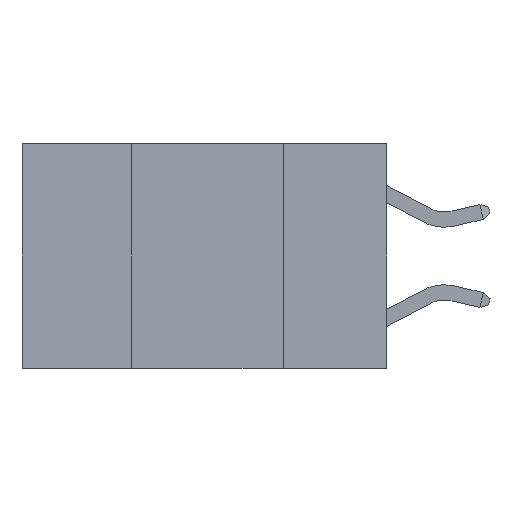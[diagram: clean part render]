
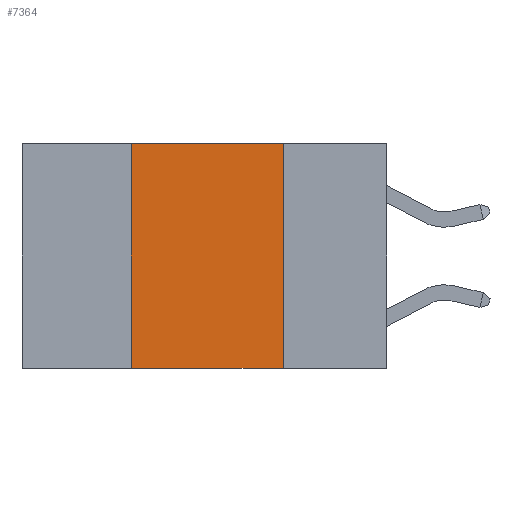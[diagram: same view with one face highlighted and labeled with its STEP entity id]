
A CAD part, left-side view. The second image highlights one B-rep face of the part: STEP entity #7364.
In plain terms, the highlighted planar face has unit normal (-1, 0, 0).
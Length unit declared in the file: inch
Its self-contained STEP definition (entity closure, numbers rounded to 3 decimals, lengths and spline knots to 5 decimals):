
#1609 = VECTOR ( 'NONE', #2965, 39.37008 ) ;
#1902 = CARTESIAN_POINT ( 'NONE',  ( 0., 0.17, 0. ) ) ;
#1964 = PLANE ( 'NONE',  #10545 ) ;
#2076 = LINE ( 'NONE', #8382, #9908 ) ;
#2579 = LINE ( 'NONE', #5825, #6420 ) ;
#2965 = DIRECTION ( 'NONE',  ( 0., 0., -1. ) ) ;
#3008 = CARTESIAN_POINT ( 'NONE',  ( 0., 0.42, 0. ) ) ;
#3349 = ORIENTED_EDGE ( 'NONE', *, *, #4575, .F. ) ;
#3635 = DIRECTION ( 'NONE',  ( 1., 0., 0. ) ) ;
#4575 = EDGE_CURVE ( 'NONE', #19919, #12928, #2579, .T. ) ;
#5216 = CARTESIAN_POINT ( 'NONE',  ( 0., 0.6, 0. ) ) ;
#5654 = VERTEX_POINT ( 'NONE', #13498 ) ;
#5825 = CARTESIAN_POINT ( 'NONE',  ( 0., 0.6, 0. ) ) ;
#6420 = VECTOR ( 'NONE', #19745, 39.37008 ) ;
#7364 = ADVANCED_FACE ( 'NONE', ( #16298 ), #1964, .F. ) ;
#8382 = CARTESIAN_POINT ( 'NONE',  ( 0., 0.6, -0.37 ) ) ;
#8672 = ORIENTED_EDGE ( 'NONE', *, *, #12689, .F. ) ;
#9908 = VECTOR ( 'NONE', #14863, 39.37008 ) ;
#10018 = DIRECTION ( 'NONE',  ( 0., 0., -1. ) ) ;
#10065 = EDGE_LOOP ( 'NONE', ( #8672, #3349, #12388, #20094 ) ) ;
#10545 = AXIS2_PLACEMENT_3D ( 'NONE', #5216, #3635, #10018 ) ;
#10714 = CARTESIAN_POINT ( 'NONE',  ( 0., 0.17, 0. ) ) ;
#11435 = EDGE_CURVE ( 'NONE', #5654, #13094, #2076, .T. ) ;
#12388 = ORIENTED_EDGE ( 'NONE', *, *, #16406, .F. ) ;
#12403 = CARTESIAN_POINT ( 'NONE',  ( 0., 0.42, 0. ) ) ;
#12689 = EDGE_CURVE ( 'NONE', #12928, #13094, #20238, .T. ) ;
#12928 = VERTEX_POINT ( 'NONE', #1902 ) ;
#13094 = VERTEX_POINT ( 'NONE', #13213 ) ;
#13213 = CARTESIAN_POINT ( 'NONE',  ( 0., 0.17, -0.37 ) ) ;
#13498 = CARTESIAN_POINT ( 'NONE',  ( 0., 0.42, -0.37 ) ) ;
#14863 = DIRECTION ( 'NONE',  ( 0., -1., 0. ) ) ;
#16298 = FACE_OUTER_BOUND ( 'NONE', #10065, .T. ) ;
#16406 = EDGE_CURVE ( 'NONE', #5654, #19919, #20143, .T. ) ;
#18335 = VECTOR ( 'NONE', #18540, 39.37008 ) ;
#18540 = DIRECTION ( 'NONE',  ( 0., 0., 1. ) ) ;
#19745 = DIRECTION ( 'NONE',  ( 0., -1., 0. ) ) ;
#19919 = VERTEX_POINT ( 'NONE', #3008 ) ;
#20094 = ORIENTED_EDGE ( 'NONE', *, *, #11435, .T. ) ;
#20143 = LINE ( 'NONE', #12403, #18335 ) ;
#20238 = LINE ( 'NONE', #10714, #1609 ) ;
